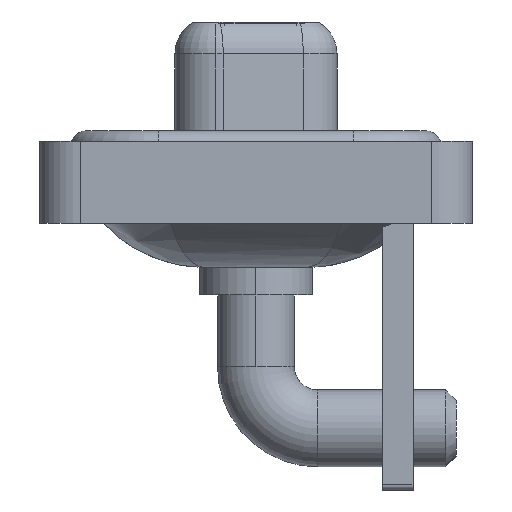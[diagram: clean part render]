
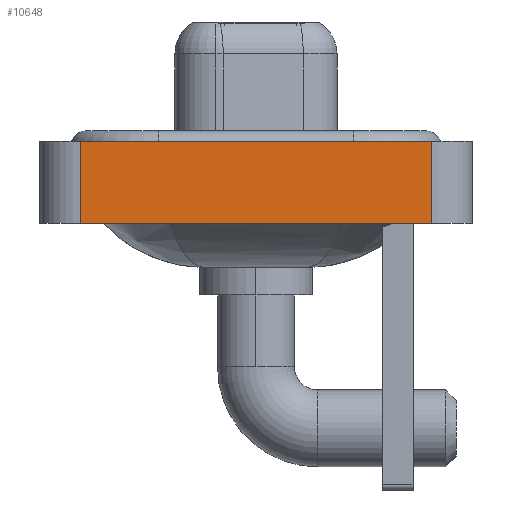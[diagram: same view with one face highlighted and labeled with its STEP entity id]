
A CAD part, left-side view. The second image highlights one B-rep face of the part: STEP entity #10648.
In plain terms, the highlighted planar face has unit normal (-1, 0, 0).
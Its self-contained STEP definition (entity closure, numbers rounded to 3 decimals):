
#304 = VECTOR ( 'NONE', #12165, 1000. ) ;
#363 = DIRECTION ( 'NONE',  ( -1., 0., 0. ) ) ;
#1076 = ORIENTED_EDGE ( 'NONE', *, *, #8437, .T. ) ;
#1295 = VECTOR ( 'NONE', #12517, 1000. ) ;
#1465 = CARTESIAN_POINT ( 'NONE',  ( -7.3, -8.55, -3.6 ) ) ;
#1724 = CARTESIAN_POINT ( 'NONE',  ( -7.3, 8.55, -3.6 ) ) ;
#2572 = DIRECTION ( 'NONE',  ( 0., -1., 0. ) ) ;
#3878 = EDGE_CURVE ( 'NONE', #15931, #8441, #9449, .T. ) ;
#4179 = PLANE ( 'NONE',  #14201 ) ;
#5768 = CARTESIAN_POINT ( 'NONE',  ( -7.3, -8.55, -3.6 ) ) ;
#5972 = ORIENTED_EDGE ( 'NONE', *, *, #9187, .T. ) ;
#7022 = DIRECTION ( 'NONE',  ( 0., 0., 1. ) ) ;
#8076 = VERTEX_POINT ( 'NONE', #1465 ) ;
#8286 = ORIENTED_EDGE ( 'NONE', *, *, #16237, .F. ) ;
#8341 = CARTESIAN_POINT ( 'NONE',  ( -7.3, -8.55, 0.4 ) ) ;
#8371 = VECTOR ( 'NONE', #7022, 1000. ) ;
#8437 = EDGE_CURVE ( 'NONE', #13500, #8076, #10882, .T. ) ;
#8441 = VERTEX_POINT ( 'NONE', #8341 ) ;
#8675 = EDGE_LOOP ( 'NONE', ( #5972, #12084, #8286, #1076 ) ) ;
#8909 = CARTESIAN_POINT ( 'NONE',  ( -7.3, 8.55, 0.4 ) ) ;
#9187 = EDGE_CURVE ( 'NONE', #8076, #8441, #15220, .T. ) ;
#9449 = LINE ( 'NONE', #16092, #304 ) ;
#10648 = ADVANCED_FACE ( 'NONE', ( #15865 ), #4179, .T. ) ;
#10882 = LINE ( 'NONE', #5768, #14849 ) ;
#11858 = DIRECTION ( 'NONE',  ( 0., 0., 1. ) ) ;
#12084 = ORIENTED_EDGE ( 'NONE', *, *, #3878, .F. ) ;
#12165 = DIRECTION ( 'NONE',  ( 0., -1., 0. ) ) ;
#12517 = DIRECTION ( 'NONE',  ( 0., 0., 1. ) ) ;
#13141 = CARTESIAN_POINT ( 'NONE',  ( -7.3, -8.55, -3.6 ) ) ;
#13387 = LINE ( 'NONE', #1724, #1295 ) ;
#13500 = VERTEX_POINT ( 'NONE', #15937 ) ;
#13933 = CARTESIAN_POINT ( 'NONE',  ( -7.3, -8.55, -3.6 ) ) ;
#14201 = AXIS2_PLACEMENT_3D ( 'NONE', #13141, #363, #11858 ) ;
#14849 = VECTOR ( 'NONE', #2572, 1000. ) ;
#15220 = LINE ( 'NONE', #13933, #8371 ) ;
#15865 = FACE_OUTER_BOUND ( 'NONE', #8675, .T. ) ;
#15931 = VERTEX_POINT ( 'NONE', #8909 ) ;
#15937 = CARTESIAN_POINT ( 'NONE',  ( -7.3, 8.55, -3.6 ) ) ;
#16092 = CARTESIAN_POINT ( 'NONE',  ( -7.3, -8.55, 0.4 ) ) ;
#16237 = EDGE_CURVE ( 'NONE', #13500, #15931, #13387, .T. ) ;
